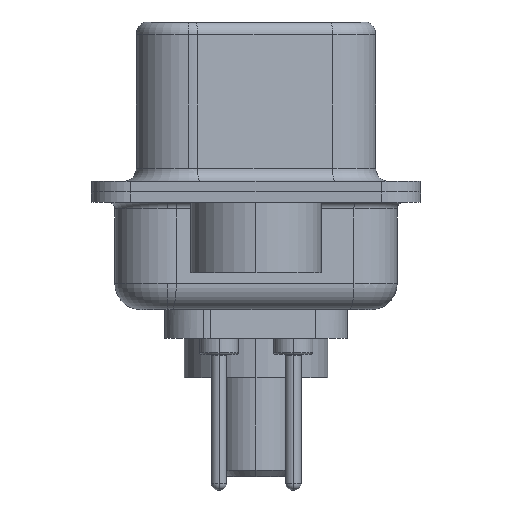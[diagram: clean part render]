
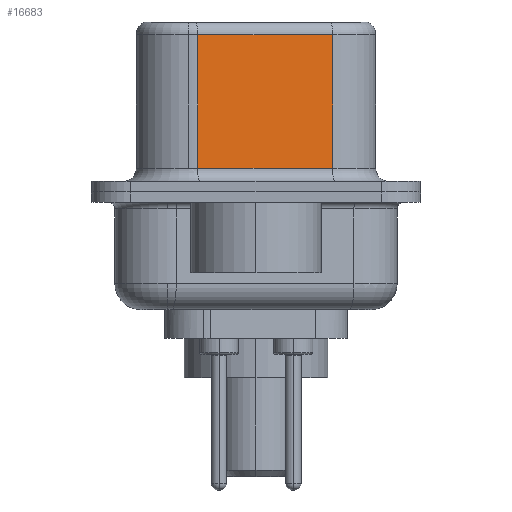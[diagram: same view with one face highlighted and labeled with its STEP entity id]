
A CAD part, left-side view. The second image highlights one B-rep face of the part: STEP entity #16683.
In plain terms, the highlighted planar face has unit normal (-0.985, -0.174, 0).
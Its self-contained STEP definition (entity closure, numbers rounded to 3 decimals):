
#502 = DIRECTION ( 'NONE',  ( -0.174, 0.985, 0. ) ) ;
#699 = CARTESIAN_POINT ( 'NONE',  ( 3.67, 2.233, 0.9 ) ) ;
#1141 = VECTOR ( 'NONE', #3871, 1000. ) ;
#1595 = LINE ( 'NONE', #5188, #1141 ) ;
#1908 = DIRECTION ( 'NONE',  ( 0., 0., -1. ) ) ;
#1972 = CARTESIAN_POINT ( 'NONE',  ( 4.58, -2.927, 6.52 ) ) ;
#2215 = LINE ( 'NONE', #1972, #8706 ) ;
#2518 = AXIS2_PLACEMENT_3D ( 'NONE', #7055, #8336, #502 ) ;
#2932 = CARTESIAN_POINT ( 'NONE',  ( 3.67, 2.233, 6.02 ) ) ;
#3349 = ORIENTED_EDGE ( 'NONE', *, *, #3900, .T. ) ;
#3513 = ORIENTED_EDGE ( 'NONE', *, *, #12969, .F. ) ;
#3871 = DIRECTION ( 'NONE',  ( 0., 0., -1. ) ) ;
#3900 = EDGE_CURVE ( 'NONE', #5886, #6494, #1595, .T. ) ;
#4129 = CARTESIAN_POINT ( 'NONE',  ( 4.58, -2.927, 0.9 ) ) ;
#5099 = EDGE_LOOP ( 'NONE', ( #3513, #15807, #3349, #7228 ) ) ;
#5188 = CARTESIAN_POINT ( 'NONE',  ( 3.67, 2.233, 6.52 ) ) ;
#5397 = FACE_OUTER_BOUND ( 'NONE', #5099, .T. ) ;
#5886 = VERTEX_POINT ( 'NONE', #2932 ) ;
#6046 = CARTESIAN_POINT ( 'NONE',  ( 4.58, -2.927, 6.02 ) ) ;
#6489 = LINE ( 'NONE', #16362, #9514 ) ;
#6494 = VERTEX_POINT ( 'NONE', #699 ) ;
#6581 = CARTESIAN_POINT ( 'NONE',  ( 4.58, -2.927, 6.02 ) ) ;
#7055 = CARTESIAN_POINT ( 'NONE',  ( 4.58, -2.927, 6.52 ) ) ;
#7228 = ORIENTED_EDGE ( 'NONE', *, *, #12136, .T. ) ;
#7392 = DIRECTION ( 'NONE',  ( 0.174, -0.985, 0. ) ) ;
#8336 = DIRECTION ( 'NONE',  ( 0.985, 0.174, 0. ) ) ;
#8706 = VECTOR ( 'NONE', #1908, 1000. ) ;
#9107 = EDGE_CURVE ( 'NONE', #10165, #5886, #9593, .T. ) ;
#9514 = VECTOR ( 'NONE', #7392, 1000. ) ;
#9593 = LINE ( 'NONE', #6046, #15571 ) ;
#9932 = DIRECTION ( 'NONE',  ( -0.174, 0.985, 0. ) ) ;
#10165 = VERTEX_POINT ( 'NONE', #6581 ) ;
#12136 = EDGE_CURVE ( 'NONE', #6494, #15179, #6489, .T. ) ;
#12969 = EDGE_CURVE ( 'NONE', #10165, #15179, #2215, .T. ) ;
#14691 = PLANE ( 'NONE',  #2518 ) ;
#15179 = VERTEX_POINT ( 'NONE', #4129 ) ;
#15571 = VECTOR ( 'NONE', #9932, 1000. ) ;
#15807 = ORIENTED_EDGE ( 'NONE', *, *, #9107, .T. ) ;
#16362 = CARTESIAN_POINT ( 'NONE',  ( 4.58, -2.927, 0.9 ) ) ;
#16683 = ADVANCED_FACE ( 'NONE', ( #5397 ), #14691, .F. ) ;
